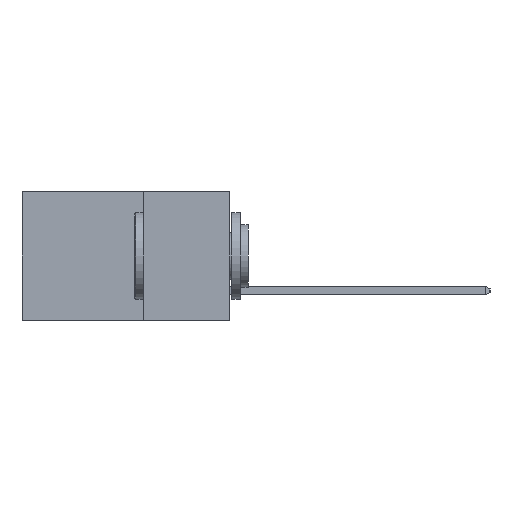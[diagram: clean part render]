
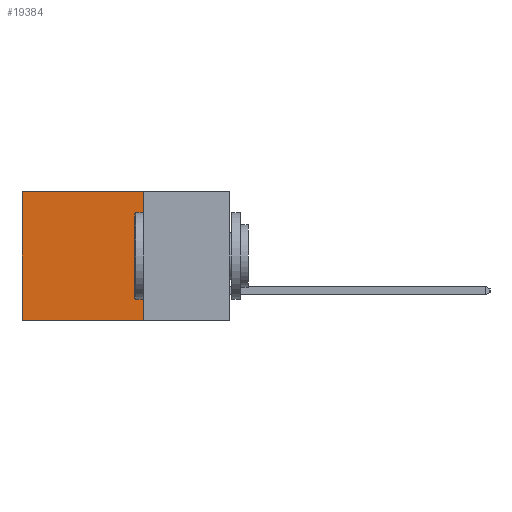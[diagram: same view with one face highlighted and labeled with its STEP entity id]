
A CAD part, left-side view. The second image highlights one B-rep face of the part: STEP entity #19384.
In plain terms, the highlighted planar face has unit normal (-1, 0, 0).
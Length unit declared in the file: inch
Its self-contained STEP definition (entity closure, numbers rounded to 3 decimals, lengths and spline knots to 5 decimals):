
#614 = DIRECTION ( 'NONE',  ( 0., 0., -1. ) ) ;
#1172 = DIRECTION ( 'NONE',  ( 0., 0., -1. ) ) ;
#1421 = ORIENTED_EDGE ( 'NONE', *, *, #9852, .F. ) ;
#1637 = ORIENTED_EDGE ( 'NONE', *, *, #22681, .T. ) ;
#2736 = CARTESIAN_POINT ( 'NONE',  ( 0.298, 0.6, 0. ) ) ;
#3651 = LINE ( 'NONE', #18778, #24833 ) ;
#4808 = FACE_OUTER_BOUND ( 'NONE', #23084, .T. ) ;
#5642 = VERTEX_POINT ( 'NONE', #11246 ) ;
#5941 = LINE ( 'NONE', #11016, #15745 ) ;
#7885 = DIRECTION ( 'NONE',  ( 0., 1., 0. ) ) ;
#8120 = DIRECTION ( 'NONE',  ( 0., 1., 0. ) ) ;
#9444 = VECTOR ( 'NONE', #8120, 39.37008 ) ;
#9852 = EDGE_CURVE ( 'NONE', #5642, #17783, #24633, .T. ) ;
#10532 = VECTOR ( 'NONE', #7885, 39.37008 ) ;
#11016 = CARTESIAN_POINT ( 'NONE',  ( 0.298, 0.6, 0. ) ) ;
#11246 = CARTESIAN_POINT ( 'NONE',  ( 0.298, 0.25, -0.37 ) ) ;
#12330 = EDGE_CURVE ( 'NONE', #23640, #5642, #3651, .T. ) ;
#12502 = DIRECTION ( 'NONE',  ( 1., 0., 0. ) ) ;
#13830 = ORIENTED_EDGE ( 'NONE', *, *, #12330, .F. ) ;
#15624 = CARTESIAN_POINT ( 'NONE',  ( 0.298, 0.25, 0. ) ) ;
#15687 = LINE ( 'NONE', #15624, #10532 ) ;
#15745 = VECTOR ( 'NONE', #22506, 39.37008 ) ;
#17743 = CARTESIAN_POINT ( 'NONE',  ( 0.298, 0.25, -0.37 ) ) ;
#17783 = VERTEX_POINT ( 'NONE', #18654 ) ;
#18427 = EDGE_CURVE ( 'NONE', #20108, #17783, #5941, .T. ) ;
#18654 = CARTESIAN_POINT ( 'NONE',  ( 0.298, 0.6, -0.37 ) ) ;
#18778 = CARTESIAN_POINT ( 'NONE',  ( 0.298, 0.25, 0. ) ) ;
#19384 = ADVANCED_FACE ( 'NONE', ( #4808 ), #20029, .F. ) ;
#19522 = AXIS2_PLACEMENT_3D ( 'NONE', #23852, #12502, #614 ) ;
#20029 = PLANE ( 'NONE',  #19522 ) ;
#20108 = VERTEX_POINT ( 'NONE', #2736 ) ;
#22506 = DIRECTION ( 'NONE',  ( 0., 0., -1. ) ) ;
#22681 = EDGE_CURVE ( 'NONE', #23640, #20108, #15687, .T. ) ;
#22850 = ORIENTED_EDGE ( 'NONE', *, *, #18427, .T. ) ;
#23084 = EDGE_LOOP ( 'NONE', ( #22850, #1421, #13830, #1637 ) ) ;
#23640 = VERTEX_POINT ( 'NONE', #24322 ) ;
#23852 = CARTESIAN_POINT ( 'NONE',  ( 0.298, 0.25, 0. ) ) ;
#24322 = CARTESIAN_POINT ( 'NONE',  ( 0.298, 0.25, 0. ) ) ;
#24633 = LINE ( 'NONE', #17743, #9444 ) ;
#24833 = VECTOR ( 'NONE', #1172, 39.37008 ) ;
